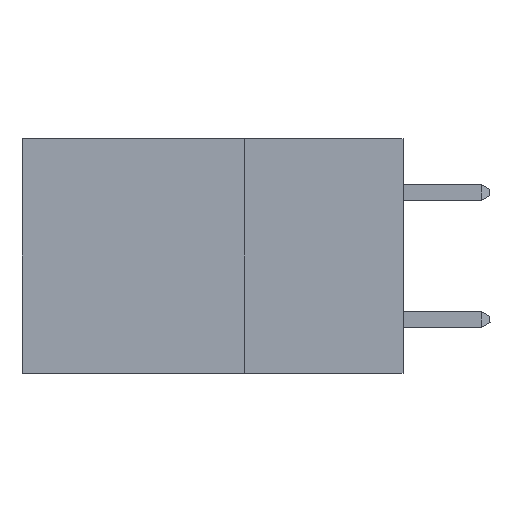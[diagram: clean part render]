
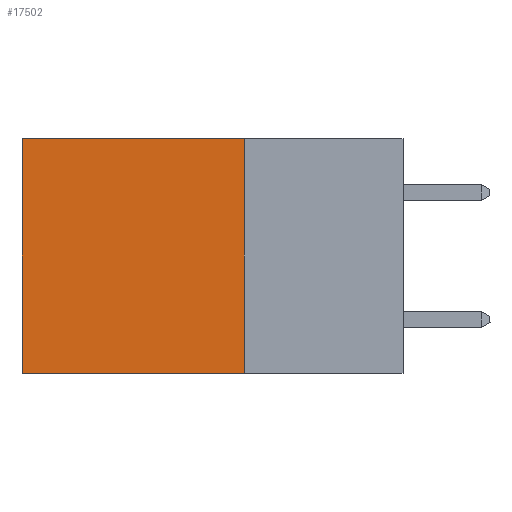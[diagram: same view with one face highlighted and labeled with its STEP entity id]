
A CAD part, left-side view. The second image highlights one B-rep face of the part: STEP entity #17502.
In plain terms, the highlighted planar face has unit normal (-1, 0, 0).
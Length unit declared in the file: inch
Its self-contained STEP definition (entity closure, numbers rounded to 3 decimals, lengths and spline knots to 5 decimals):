
#783 = VECTOR ( 'NONE', #15998, 39.37008 ) ;
#1705 = DIRECTION ( 'NONE',  ( 1., 0., 0. ) ) ;
#2018 = VECTOR ( 'NONE', #18735, 39.37008 ) ;
#2828 = VECTOR ( 'NONE', #9709, 39.37008 ) ;
#2974 = ORIENTED_EDGE ( 'NONE', *, *, #4734, .F. ) ;
#3552 = ORIENTED_EDGE ( 'NONE', *, *, #9893, .T. ) ;
#3761 = VERTEX_POINT ( 'NONE', #19727 ) ;
#4241 = LINE ( 'NONE', #22096, #783 ) ;
#4691 = VERTEX_POINT ( 'NONE', #26130 ) ;
#4734 = EDGE_CURVE ( 'NONE', #4691, #15892, #13652, .T. ) ;
#6762 = FACE_OUTER_BOUND ( 'NONE', #8419, .T. ) ;
#8419 = EDGE_LOOP ( 'NONE', ( #3552, #2974, #25251, #14156 ) ) ;
#9051 = DIRECTION ( 'NONE',  ( 0., 1., 0. ) ) ;
#9242 = CARTESIAN_POINT ( 'NONE',  ( 0.2875, 0.25, 0. ) ) ;
#9709 = DIRECTION ( 'NONE',  ( 0., 0., -1. ) ) ;
#9893 = EDGE_CURVE ( 'NONE', #3761, #15892, #10119, .T. ) ;
#10119 = LINE ( 'NONE', #17881, #2828 ) ;
#10330 = CARTESIAN_POINT ( 'NONE',  ( 0.2875, 0.6, -0.37 ) ) ;
#13652 = LINE ( 'NONE', #15598, #25768 ) ;
#14156 = ORIENTED_EDGE ( 'NONE', *, *, #17597, .T. ) ;
#15598 = CARTESIAN_POINT ( 'NONE',  ( 0.2875, 0.25, -0.37 ) ) ;
#15892 = VERTEX_POINT ( 'NONE', #10330 ) ;
#15998 = DIRECTION ( 'NONE',  ( 0., 0., -1. ) ) ;
#16996 = DIRECTION ( 'NONE',  ( 0., 0., -1. ) ) ;
#17130 = EDGE_CURVE ( 'NONE', #21241, #4691, #4241, .T. ) ;
#17502 = ADVANCED_FACE ( 'NONE', ( #6762 ), #25680, .F. ) ;
#17597 = EDGE_CURVE ( 'NONE', #21241, #3761, #22469, .T. ) ;
#17881 = CARTESIAN_POINT ( 'NONE',  ( 0.2875, 0.6, 0. ) ) ;
#18735 = DIRECTION ( 'NONE',  ( 0., 1., 0. ) ) ;
#19727 = CARTESIAN_POINT ( 'NONE',  ( 0.2875, 0.6, 0. ) ) ;
#21241 = VERTEX_POINT ( 'NONE', #9242 ) ;
#21898 = AXIS2_PLACEMENT_3D ( 'NONE', #23393, #1705, #16996 ) ;
#22096 = CARTESIAN_POINT ( 'NONE',  ( 0.2875, 0.25, 0. ) ) ;
#22469 = LINE ( 'NONE', #25018, #2018 ) ;
#23393 = CARTESIAN_POINT ( 'NONE',  ( 0.2875, 0.25, 0. ) ) ;
#25018 = CARTESIAN_POINT ( 'NONE',  ( 0.2875, 0.25, 0. ) ) ;
#25251 = ORIENTED_EDGE ( 'NONE', *, *, #17130, .F. ) ;
#25680 = PLANE ( 'NONE',  #21898 ) ;
#25768 = VECTOR ( 'NONE', #9051, 39.37008 ) ;
#26130 = CARTESIAN_POINT ( 'NONE',  ( 0.2875, 0.25, -0.37 ) ) ;
